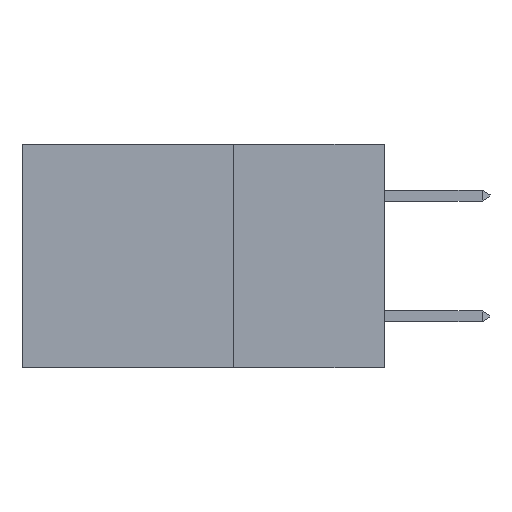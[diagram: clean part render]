
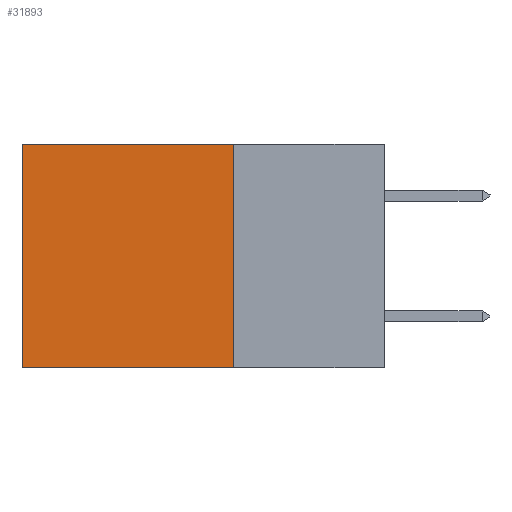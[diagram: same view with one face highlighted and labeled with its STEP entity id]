
A CAD part, left-side view. The second image highlights one B-rep face of the part: STEP entity #31893.
In plain terms, the highlighted planar face has unit normal (-1, 0, 0).
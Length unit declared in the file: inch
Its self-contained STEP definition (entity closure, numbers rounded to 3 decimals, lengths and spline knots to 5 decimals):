
#5432 = VECTOR ( 'NONE', #26914, 39.37008 ) ;
#5819 = VECTOR ( 'NONE', #11153, 39.37008 ) ;
#6328 = LINE ( 'NONE', #30616, #5819 ) ;
#8090 = VERTEX_POINT ( 'NONE', #35094 ) ;
#8841 = EDGE_CURVE ( 'NONE', #22403, #22139, #34491, .T. ) ;
#9295 = VERTEX_POINT ( 'NONE', #30692 ) ;
#11153 = DIRECTION ( 'NONE',  ( 0., 1., 0. ) ) ;
#11395 = EDGE_CURVE ( 'NONE', #9295, #22139, #36719, .T. ) ;
#11430 = LINE ( 'NONE', #14446, #5432 ) ;
#14446 = CARTESIAN_POINT ( 'NONE',  ( 0.2875, 0.25, 0. ) ) ;
#15204 = PLANE ( 'NONE',  #33563 ) ;
#15618 = ORIENTED_EDGE ( 'NONE', *, *, #8841, .T. ) ;
#15879 = EDGE_LOOP ( 'NONE', ( #15618, #21915, #17121, #34021 ) ) ;
#17121 = ORIENTED_EDGE ( 'NONE', *, *, #37888, .F. ) ;
#18247 = DIRECTION ( 'NONE',  ( 0., 0., -1. ) ) ;
#19514 = FACE_OUTER_BOUND ( 'NONE', #15879, .T. ) ;
#20190 = CARTESIAN_POINT ( 'NONE',  ( 0.2875, 0.25, -0.37 ) ) ;
#21915 = ORIENTED_EDGE ( 'NONE', *, *, #11395, .F. ) ;
#22139 = VERTEX_POINT ( 'NONE', #23658 ) ;
#22403 = VERTEX_POINT ( 'NONE', #31762 ) ;
#23658 = CARTESIAN_POINT ( 'NONE',  ( 0.2875, 0.6, -0.37 ) ) ;
#25509 = DIRECTION ( 'NONE',  ( 0., 0., -1. ) ) ;
#26285 = EDGE_CURVE ( 'NONE', #8090, #22403, #6328, .T. ) ;
#26914 = DIRECTION ( 'NONE',  ( 0., 0., -1. ) ) ;
#28652 = CARTESIAN_POINT ( 'NONE',  ( 0.2875, 0.6, 0. ) ) ;
#30616 = CARTESIAN_POINT ( 'NONE',  ( 0.2875, 0.25, 0. ) ) ;
#30692 = CARTESIAN_POINT ( 'NONE',  ( 0.2875, 0.25, -0.37 ) ) ;
#30796 = CARTESIAN_POINT ( 'NONE',  ( 0.2875, 0.25, 0. ) ) ;
#31762 = CARTESIAN_POINT ( 'NONE',  ( 0.2875, 0.6, 0. ) ) ;
#31893 = ADVANCED_FACE ( 'NONE', ( #19514 ), #15204, .F. ) ;
#33563 = AXIS2_PLACEMENT_3D ( 'NONE', #30796, #37012, #18247 ) ;
#34021 = ORIENTED_EDGE ( 'NONE', *, *, #26285, .T. ) ;
#34491 = LINE ( 'NONE', #28652, #36661 ) ;
#35094 = CARTESIAN_POINT ( 'NONE',  ( 0.2875, 0.25, 0. ) ) ;
#36661 = VECTOR ( 'NONE', #25509, 39.37008 ) ;
#36719 = LINE ( 'NONE', #20190, #37207 ) ;
#37012 = DIRECTION ( 'NONE',  ( 1., 0., 0. ) ) ;
#37207 = VECTOR ( 'NONE', #39898, 39.37008 ) ;
#37888 = EDGE_CURVE ( 'NONE', #8090, #9295, #11430, .T. ) ;
#39898 = DIRECTION ( 'NONE',  ( 0., 1., 0. ) ) ;
